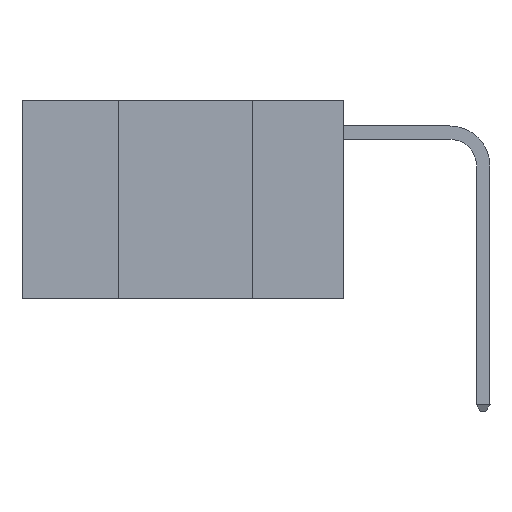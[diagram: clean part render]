
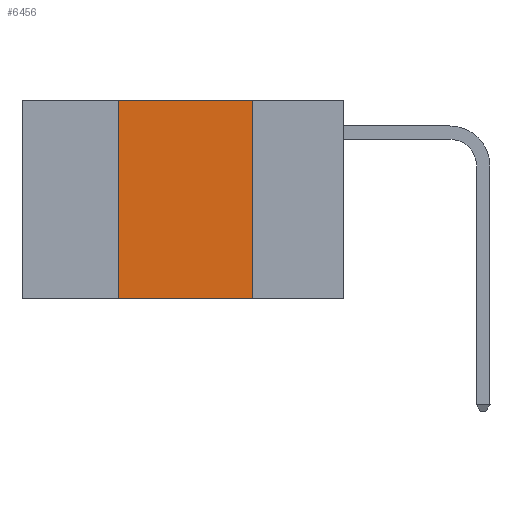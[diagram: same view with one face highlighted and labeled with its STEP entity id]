
A CAD part, left-side view. The second image highlights one B-rep face of the part: STEP entity #6456.
In plain terms, the highlighted planar face has unit normal (-1, 0, 0).
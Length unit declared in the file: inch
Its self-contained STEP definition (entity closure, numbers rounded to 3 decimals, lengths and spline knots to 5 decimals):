
#128 = VERTEX_POINT ( 'NONE', #3118 ) ;
#201 = VERTEX_POINT ( 'NONE', #8298 ) ;
#212 = VECTOR ( 'NONE', #3460, 39.37008 ) ;
#343 = EDGE_CURVE ( 'NONE', #128, #201, #12970, .T. ) ;
#390 = DIRECTION ( 'NONE',  ( 0., 0., -1. ) ) ;
#2287 = CARTESIAN_POINT ( 'NONE',  ( 0., 0.6, -0.37 ) ) ;
#2328 = ORIENTED_EDGE ( 'NONE', *, *, #3968, .T. ) ;
#2696 = VECTOR ( 'NONE', #10240, 39.37008 ) ;
#2847 = ORIENTED_EDGE ( 'NONE', *, *, #5882, .F. ) ;
#3118 = CARTESIAN_POINT ( 'NONE',  ( 0., 0.42, -0.37 ) ) ;
#3311 = LINE ( 'NONE', #2287, #212 ) ;
#3460 = DIRECTION ( 'NONE',  ( 0., -1., 0. ) ) ;
#3801 = CARTESIAN_POINT ( 'NONE',  ( 0., 0.17, 0. ) ) ;
#3968 = EDGE_CURVE ( 'NONE', #128, #9720, #3311, .T. ) ;
#4945 = FACE_OUTER_BOUND ( 'NONE', #7874, .T. ) ;
#5878 = PLANE ( 'NONE',  #10320 ) ;
#5882 = EDGE_CURVE ( 'NONE', #201, #7755, #13921, .T. ) ;
#5885 = VECTOR ( 'NONE', #6190, 39.37008 ) ;
#6190 = DIRECTION ( 'NONE',  ( 0., 0., 1. ) ) ;
#6456 = ADVANCED_FACE ( 'NONE', ( #4945 ), #5878, .F. ) ;
#6661 = CARTESIAN_POINT ( 'NONE',  ( 0., 0.17, 0. ) ) ;
#7755 = VERTEX_POINT ( 'NONE', #3801 ) ;
#7874 = EDGE_LOOP ( 'NONE', ( #9089, #2847, #9760, #2328 ) ) ;
#8298 = CARTESIAN_POINT ( 'NONE',  ( 0., 0.42, 0. ) ) ;
#9089 = ORIENTED_EDGE ( 'NONE', *, *, #14206, .F. ) ;
#9720 = VERTEX_POINT ( 'NONE', #11169 ) ;
#9760 = ORIENTED_EDGE ( 'NONE', *, *, #343, .F. ) ;
#9769 = CARTESIAN_POINT ( 'NONE',  ( 0., 0.42, 0. ) ) ;
#9954 = LINE ( 'NONE', #6661, #2696 ) ;
#10240 = DIRECTION ( 'NONE',  ( 0., 0., -1. ) ) ;
#10320 = AXIS2_PLACEMENT_3D ( 'NONE', #10350, #12675, #390 ) ;
#10350 = CARTESIAN_POINT ( 'NONE',  ( 0., 0.6, 0. ) ) ;
#10513 = CARTESIAN_POINT ( 'NONE',  ( 0., 0.6, 0. ) ) ;
#11169 = CARTESIAN_POINT ( 'NONE',  ( 0., 0.17, -0.37 ) ) ;
#11603 = VECTOR ( 'NONE', #13982, 39.37008 ) ;
#12675 = DIRECTION ( 'NONE',  ( 1., 0., 0. ) ) ;
#12970 = LINE ( 'NONE', #9769, #5885 ) ;
#13921 = LINE ( 'NONE', #10513, #11603 ) ;
#13982 = DIRECTION ( 'NONE',  ( 0., -1., 0. ) ) ;
#14206 = EDGE_CURVE ( 'NONE', #7755, #9720, #9954, .T. ) ;
